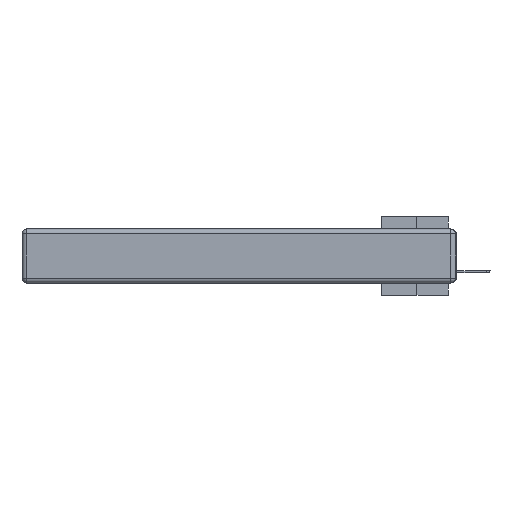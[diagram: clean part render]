
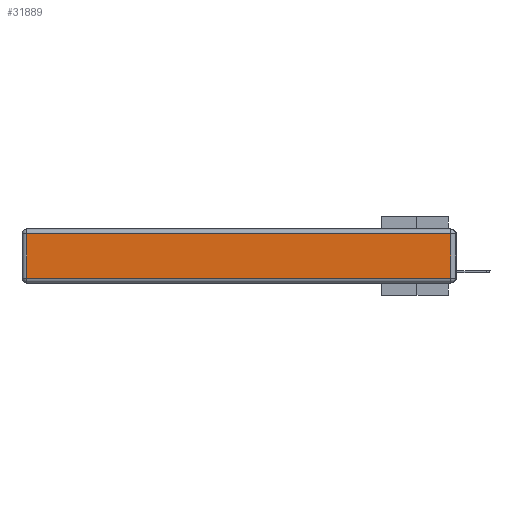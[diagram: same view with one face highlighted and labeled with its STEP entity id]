
A CAD part, left-side view. The second image highlights one B-rep face of the part: STEP entity #31889.
In plain terms, the highlighted planar face has unit normal (-1, 0, 0).
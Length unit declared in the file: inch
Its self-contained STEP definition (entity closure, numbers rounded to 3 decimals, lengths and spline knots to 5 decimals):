
#186 = CARTESIAN_POINT ( 'NONE',  ( 0., 0., -0.343 ) ) ;
#2270 = DIRECTION ( 'NONE',  ( 0., 1., 0. ) ) ;
#3037 = DIRECTION ( 'NONE',  ( -1., 0., 0. ) ) ;
#5537 = ORIENTED_EDGE ( 'NONE', *, *, #13830, .T. ) ;
#6452 = PLANE ( 'NONE',  #39374 ) ;
#6982 = VERTEX_POINT ( 'NONE', #16176 ) ;
#7185 = CARTESIAN_POINT ( 'NONE',  ( 0., 0.03, -0.343 ) ) ;
#7504 = VERTEX_POINT ( 'NONE', #12798 ) ;
#7778 = CARTESIAN_POINT ( 'NONE',  ( 0., 0., -0.313 ) ) ;
#8872 = EDGE_CURVE ( 'NONE', #7504, #28877, #24992, .T. ) ;
#10710 = LINE ( 'NONE', #30624, #22362 ) ;
#12798 = CARTESIAN_POINT ( 'NONE',  ( 0., 2.72, -0.313 ) ) ;
#13830 = EDGE_CURVE ( 'NONE', #6982, #7504, #10710, .T. ) ;
#14443 = ORIENTED_EDGE ( 'NONE', *, *, #19073, .T. ) ;
#14854 = EDGE_LOOP ( 'NONE', ( #17971, #14443, #38432, #5537 ) ) ;
#16176 = CARTESIAN_POINT ( 'NONE',  ( 0., 2.72, -0.03 ) ) ;
#16235 = CARTESIAN_POINT ( 'NONE',  ( 0., 0.03, -0.313 ) ) ;
#16913 = EDGE_CURVE ( 'NONE', #17209, #6982, #30338, .T. ) ;
#17209 = VERTEX_POINT ( 'NONE', #37409 ) ;
#17752 = FACE_OUTER_BOUND ( 'NONE', #14854, .T. ) ;
#17971 = ORIENTED_EDGE ( 'NONE', *, *, #8872, .T. ) ;
#19073 = EDGE_CURVE ( 'NONE', #28877, #17209, #36971, .T. ) ;
#19654 = CARTESIAN_POINT ( 'NONE',  ( 0., 2.75, -0.03 ) ) ;
#21061 = VECTOR ( 'NONE', #38823, 39.37008 ) ;
#21959 = VECTOR ( 'NONE', #31631, 39.37008 ) ;
#22362 = VECTOR ( 'NONE', #36140, 39.37008 ) ;
#24527 = DIRECTION ( 'NONE',  ( 0., 0., 1. ) ) ;
#24992 = LINE ( 'NONE', #7778, #21061 ) ;
#28877 = VERTEX_POINT ( 'NONE', #16235 ) ;
#30338 = LINE ( 'NONE', #19654, #39443 ) ;
#30624 = CARTESIAN_POINT ( 'NONE',  ( 0., 2.72, -0.343 ) ) ;
#31631 = DIRECTION ( 'NONE',  ( 0., 0., 1. ) ) ;
#31889 = ADVANCED_FACE ( 'NONE', ( #17752 ), #6452, .T. ) ;
#36140 = DIRECTION ( 'NONE',  ( 0., 0., -1. ) ) ;
#36971 = LINE ( 'NONE', #7185, #21959 ) ;
#37409 = CARTESIAN_POINT ( 'NONE',  ( 0., 0.03, -0.03 ) ) ;
#38432 = ORIENTED_EDGE ( 'NONE', *, *, #16913, .T. ) ;
#38823 = DIRECTION ( 'NONE',  ( 0., -1., 0. ) ) ;
#39374 = AXIS2_PLACEMENT_3D ( 'NONE', #186, #3037, #24527 ) ;
#39443 = VECTOR ( 'NONE', #2270, 39.37008 ) ;
